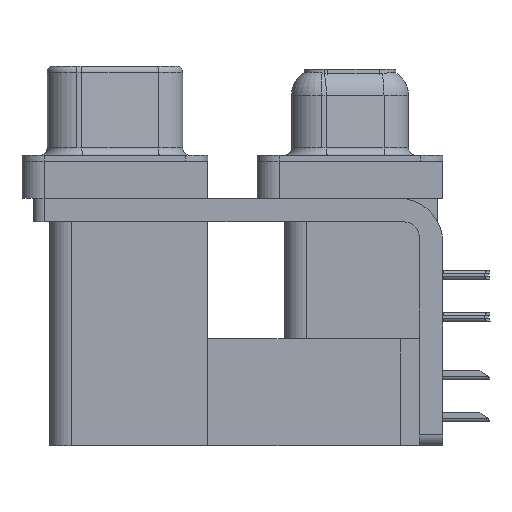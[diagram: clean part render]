
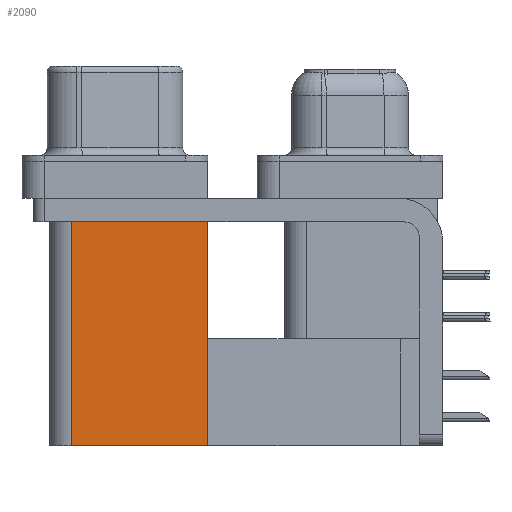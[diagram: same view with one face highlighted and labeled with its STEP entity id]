
A CAD part, left-side view. The second image highlights one B-rep face of the part: STEP entity #2090.
In plain terms, the highlighted planar face has unit normal (-1, 0, 0).
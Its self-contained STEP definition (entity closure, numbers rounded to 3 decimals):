
#2090 = ADVANCED_FACE ( 'NONE', ( #24999 ), #18117, .F. ) ;
#4113 = CARTESIAN_POINT ( 'NONE',  ( 3.765, 9.6, -19.2 ) ) ;
#5161 = LINE ( 'NONE', #38997, #19172 ) ;
#5399 = EDGE_CURVE ( 'NONE', #38155, #16523, #17045, .T. ) ;
#7760 = EDGE_LOOP ( 'NONE', ( #40854, #8704, #11803, #13011 ) ) ;
#8704 = ORIENTED_EDGE ( 'NONE', *, *, #5399, .F. ) ;
#9397 = VERTEX_POINT ( 'NONE', #37808 ) ;
#10664 = CARTESIAN_POINT ( 'NONE',  ( 3.765, 18.8, -2.5 ) ) ;
#11643 = VECTOR ( 'NONE', #36664, 1000. ) ;
#11803 = ORIENTED_EDGE ( 'NONE', *, *, #34422, .F. ) ;
#12605 = DIRECTION ( 'NONE',  ( 0., 0., 1. ) ) ;
#12834 = LINE ( 'NONE', #23056, #11643 ) ;
#13011 = ORIENTED_EDGE ( 'NONE', *, *, #23715, .T. ) ;
#15755 = VERTEX_POINT ( 'NONE', #17452 ) ;
#16523 = VERTEX_POINT ( 'NONE', #10664 ) ;
#16756 = CARTESIAN_POINT ( 'NONE',  ( 3.765, 9.6, -2.5 ) ) ;
#17045 = LINE ( 'NONE', #30640, #21472 ) ;
#17433 = DIRECTION ( 'NONE',  ( 0., 1., 0. ) ) ;
#17452 = CARTESIAN_POINT ( 'NONE',  ( 3.765, 9.6, -19.2 ) ) ;
#18117 = PLANE ( 'NONE',  #30752 ) ;
#19172 = VECTOR ( 'NONE', #32764, 1000. ) ;
#21472 = VECTOR ( 'NONE', #12605, 1000. ) ;
#22181 = EDGE_CURVE ( 'NONE', #9397, #16523, #33480, .T. ) ;
#23056 = CARTESIAN_POINT ( 'NONE',  ( 3.765, 9.6, -19.2 ) ) ;
#23715 = EDGE_CURVE ( 'NONE', #15755, #9397, #12834, .T. ) ;
#24351 = VECTOR ( 'NONE', #17433, 1000. ) ;
#24999 = FACE_OUTER_BOUND ( 'NONE', #7760, .T. ) ;
#30640 = CARTESIAN_POINT ( 'NONE',  ( 3.765, 18.8, -19.2 ) ) ;
#30752 = AXIS2_PLACEMENT_3D ( 'NONE', #4113, #31698, #38618 ) ;
#31698 = DIRECTION ( 'NONE',  ( 1., 0., 0. ) ) ;
#32764 = DIRECTION ( 'NONE',  ( 0., 1., 0. ) ) ;
#33480 = LINE ( 'NONE', #16756, #24351 ) ;
#34422 = EDGE_CURVE ( 'NONE', #15755, #38155, #5161, .T. ) ;
#36664 = DIRECTION ( 'NONE',  ( 0., 0., 1. ) ) ;
#37808 = CARTESIAN_POINT ( 'NONE',  ( 3.765, 9.6, -2.5 ) ) ;
#38155 = VERTEX_POINT ( 'NONE', #43031 ) ;
#38618 = DIRECTION ( 'NONE',  ( 0., 0., -1. ) ) ;
#38997 = CARTESIAN_POINT ( 'NONE',  ( 3.765, 9.6, -19.2 ) ) ;
#40854 = ORIENTED_EDGE ( 'NONE', *, *, #22181, .T. ) ;
#43031 = CARTESIAN_POINT ( 'NONE',  ( 3.765, 18.8, -19.2 ) ) ;
